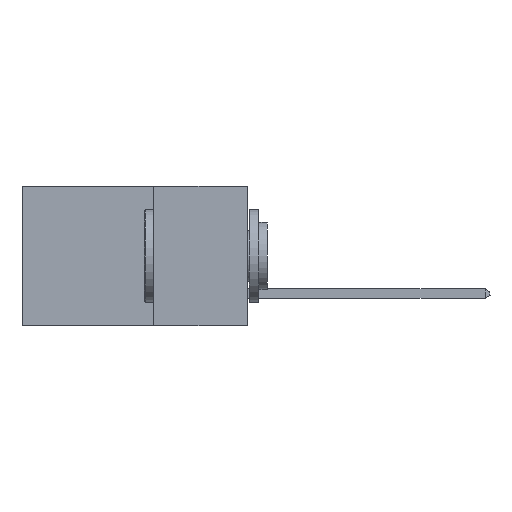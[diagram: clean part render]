
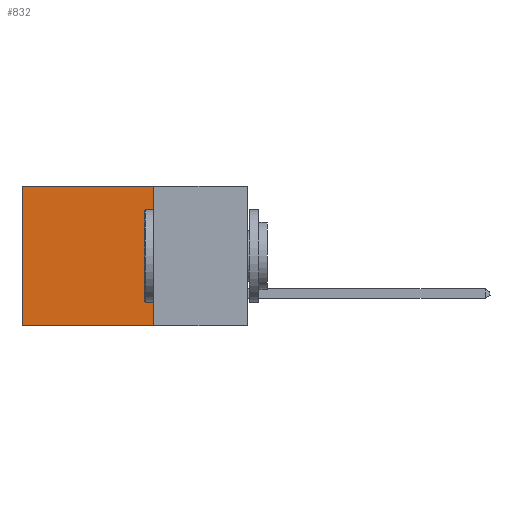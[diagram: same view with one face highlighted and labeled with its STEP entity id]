
A CAD part, left-side view. The second image highlights one B-rep face of the part: STEP entity #832.
In plain terms, the highlighted planar face has unit normal (-1, 0, 0).
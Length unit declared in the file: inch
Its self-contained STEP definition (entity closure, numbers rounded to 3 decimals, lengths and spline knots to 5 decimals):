
#316 = VECTOR ( 'NONE', #20647, 39.37008 ) ;
#832 = ADVANCED_FACE ( 'NONE', ( #15828 ), #3683, .F. ) ;
#907 = EDGE_CURVE ( 'NONE', #17207, #3297, #12918, .T. ) ;
#1466 = CARTESIAN_POINT ( 'NONE',  ( 0.298, 0.6, -0.37 ) ) ;
#1781 = EDGE_CURVE ( 'NONE', #17207, #22195, #7742, .T. ) ;
#1866 = DIRECTION ( 'NONE',  ( 0., 0., -1. ) ) ;
#2460 = LINE ( 'NONE', #12972, #11907 ) ;
#2733 = AXIS2_PLACEMENT_3D ( 'NONE', #26724, #11191, #1866 ) ;
#3297 = VERTEX_POINT ( 'NONE', #13375 ) ;
#3683 = PLANE ( 'NONE',  #2733 ) ;
#4384 = ORIENTED_EDGE ( 'NONE', *, *, #4980, .T. ) ;
#4980 = EDGE_CURVE ( 'NONE', #3297, #22609, #2460, .T. ) ;
#5101 = EDGE_CURVE ( 'NONE', #22195, #22609, #17357, .T. ) ;
#7742 = LINE ( 'NONE', #20619, #11725 ) ;
#8780 = ORIENTED_EDGE ( 'NONE', *, *, #907, .T. ) ;
#8862 = CARTESIAN_POINT ( 'NONE',  ( 0.298, 0.25, 0. ) ) ;
#11191 = DIRECTION ( 'NONE',  ( 1., 0., 0. ) ) ;
#11725 = VECTOR ( 'NONE', #22744, 39.37008 ) ;
#11907 = VECTOR ( 'NONE', #29184, 39.37008 ) ;
#12918 = LINE ( 'NONE', #8862, #17611 ) ;
#12972 = CARTESIAN_POINT ( 'NONE',  ( 0.298, 0.6, 0. ) ) ;
#13375 = CARTESIAN_POINT ( 'NONE',  ( 0.298, 0.6, 0. ) ) ;
#15828 = FACE_OUTER_BOUND ( 'NONE', #19438, .T. ) ;
#17207 = VERTEX_POINT ( 'NONE', #22270 ) ;
#17357 = LINE ( 'NONE', #25107, #316 ) ;
#17611 = VECTOR ( 'NONE', #29471, 39.37008 ) ;
#17715 = ORIENTED_EDGE ( 'NONE', *, *, #1781, .F. ) ;
#18444 = ORIENTED_EDGE ( 'NONE', *, *, #5101, .F. ) ;
#19438 = EDGE_LOOP ( 'NONE', ( #4384, #18444, #17715, #8780 ) ) ;
#20619 = CARTESIAN_POINT ( 'NONE',  ( 0.298, 0.25, 0. ) ) ;
#20647 = DIRECTION ( 'NONE',  ( 0., 1., 0. ) ) ;
#20865 = CARTESIAN_POINT ( 'NONE',  ( 0.298, 0.25, -0.37 ) ) ;
#22195 = VERTEX_POINT ( 'NONE', #20865 ) ;
#22270 = CARTESIAN_POINT ( 'NONE',  ( 0.298, 0.25, 0. ) ) ;
#22609 = VERTEX_POINT ( 'NONE', #1466 ) ;
#22744 = DIRECTION ( 'NONE',  ( 0., 0., -1. ) ) ;
#25107 = CARTESIAN_POINT ( 'NONE',  ( 0.298, 0.25, -0.37 ) ) ;
#26724 = CARTESIAN_POINT ( 'NONE',  ( 0.298, 0.25, 0. ) ) ;
#29184 = DIRECTION ( 'NONE',  ( 0., 0., -1. ) ) ;
#29471 = DIRECTION ( 'NONE',  ( 0., 1., 0. ) ) ;
